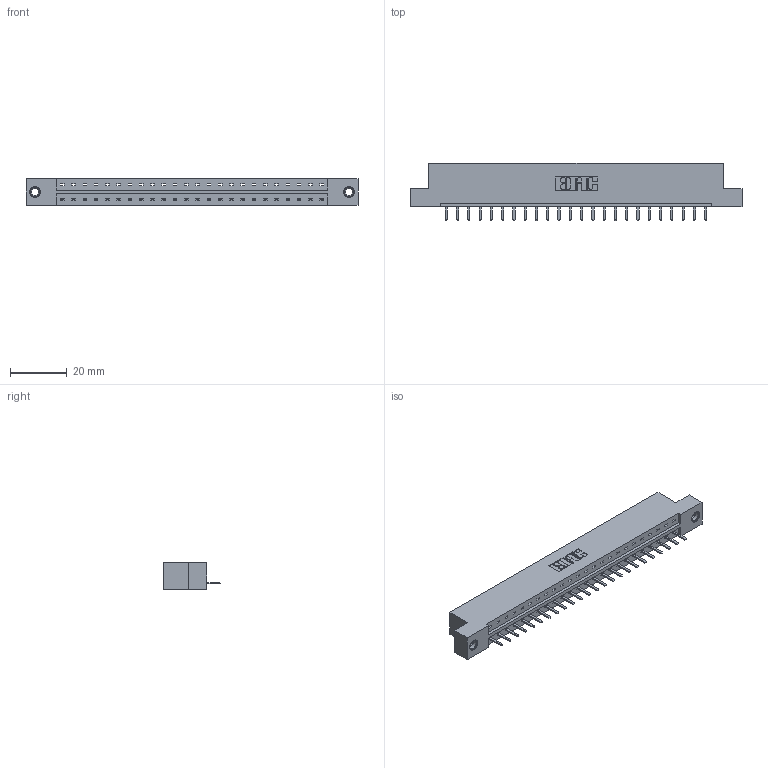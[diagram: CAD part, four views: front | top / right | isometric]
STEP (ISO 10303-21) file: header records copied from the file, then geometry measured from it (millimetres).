
FILE_DESCRIPTION (( 'STEP AP203' ), '1' );
FILE_NAME ('333-024-520-107.STEP', '2018-08-02T04:05:44', ( '' ), ( '' ), 'SwSTEP 2.0', 'SolidWorks 2016', '' );
FILE_SCHEMA (( 'CONFIG_CONTROL_DESIGN' ));
Length unit declared in the file: inch
Products named in the file (4): 345-292-001_345-293-120; 345-250-001_345-250-005-103; 333-024-520-107; 333 Part_Flush - .156 Dia - TI
Assembly tree (27 placements, depth 2):
  333-024-520-107
    333 Part_Flush - .156 Dia - TI
    345-292-001_345-293-120  x24
    345-250-001_345-250-005-103  x2
Bounding box: 116.64 x 20.02 x 9.4 mm (x, y, z)
Volume: 11499.6 mm3; surface area: 12119.9 mm2
Topology: 27 solids, 27 shells, 1662 faces, 4863 edges, 3170 vertices
Faces by surface type: plane 1158, cylinder 488, cone 12, torus 4
Entity records: 18300 total; most frequent: CARTESIAN_POINT 3153, ORIENTED_EDGE 3094, DIRECTION 2717, EDGE_CURVE 1547, VECTOR 1395, LINE 1395, VERTEX_POINT 1024, AXIS2_PLACEMENT_3D 661
